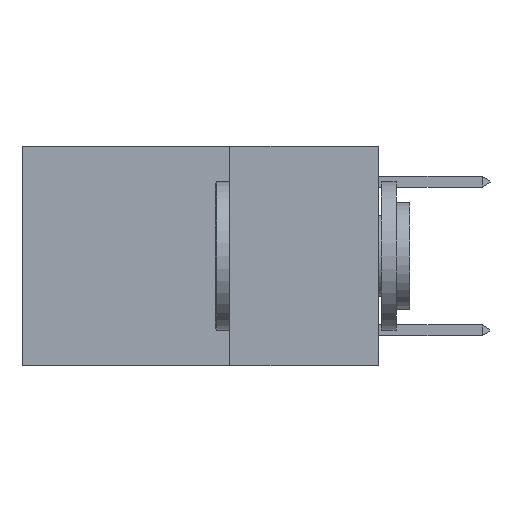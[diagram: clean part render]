
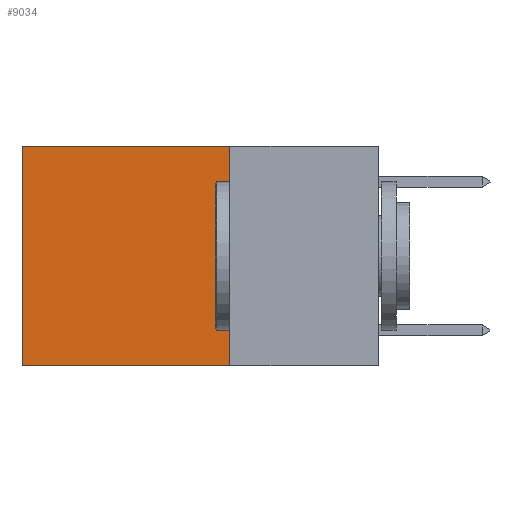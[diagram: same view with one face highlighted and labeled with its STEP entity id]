
A CAD part, left-side view. The second image highlights one B-rep face of the part: STEP entity #9034.
In plain terms, the highlighted planar face has unit normal (-1, 0, 0).
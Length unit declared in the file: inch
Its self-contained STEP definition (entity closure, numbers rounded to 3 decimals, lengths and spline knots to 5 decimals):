
#34 = EDGE_LOOP ( 'NONE', ( #12272, #21927, #20050, #18828 ) ) ;
#1859 = EDGE_CURVE ( 'NONE', #19730, #19976, #15999, .T. ) ;
#3549 = CARTESIAN_POINT ( 'NONE',  ( 0.2625, 0.25, 0. ) ) ;
#3548 = VECTOR ( 'NONE', #12937, 39.37008 ) ;
#3573 = VECTOR ( 'NONE', #8988, 39.37008 ) ;
#3718 = CARTESIAN_POINT ( 'NONE',  ( 0.2625, 0.25, -0.37 ) ) ;
#5790 = CARTESIAN_POINT ( 'NONE',  ( 0.2625, 0.25, -0.37 ) ) ;
#6037 = EDGE_CURVE ( 'NONE', #19730, #17663, #15828, .T. ) ;
#6573 = LINE ( 'NONE', #5790, #3573 ) ;
#7294 = CARTESIAN_POINT ( 'NONE',  ( 0.2625, 0.25, 0. ) ) ;
#7541 = CARTESIAN_POINT ( 'NONE',  ( 0.2625, 0.6, 0. ) ) ;
#8988 = DIRECTION ( 'NONE',  ( 0., 1., 0. ) ) ;
#9015 = LINE ( 'NONE', #9430, #3548 ) ;
#9034 = ADVANCED_FACE ( 'NONE', ( #9570 ), #20997, .F. ) ;
#9430 = CARTESIAN_POINT ( 'NONE',  ( 0.2625, 0.6, 0. ) ) ;
#9570 = FACE_OUTER_BOUND ( 'NONE', #34, .T. ) ;
#9741 = CARTESIAN_POINT ( 'NONE',  ( 0.2625, 0.6, -0.37 ) ) ;
#10288 = EDGE_CURVE ( 'NONE', #17663, #16092, #9015, .T. ) ;
#10631 = DIRECTION ( 'NONE',  ( 0., 0., -1. ) ) ;
#11020 = DIRECTION ( 'NONE',  ( 0., 1., 0. ) ) ;
#11239 = VECTOR ( 'NONE', #11020, 39.37008 ) ;
#12200 = DIRECTION ( 'NONE',  ( 0., 0., -1. ) ) ;
#12272 = ORIENTED_EDGE ( 'NONE', *, *, #10288, .T. ) ;
#12937 = DIRECTION ( 'NONE',  ( 0., 0., -1. ) ) ;
#13463 = CARTESIAN_POINT ( 'NONE',  ( 0.2625, 0.25, 0. ) ) ;
#14540 = AXIS2_PLACEMENT_3D ( 'NONE', #3549, #17423, #10631 ) ;
#15828 = LINE ( 'NONE', #7294, #11239 ) ;
#15999 = LINE ( 'NONE', #18783, #16214 ) ;
#16092 = VERTEX_POINT ( 'NONE', #9741 ) ;
#16214 = VECTOR ( 'NONE', #12200, 39.37008 ) ;
#17423 = DIRECTION ( 'NONE',  ( 1., 0., 0. ) ) ;
#17663 = VERTEX_POINT ( 'NONE', #7541 ) ;
#18783 = CARTESIAN_POINT ( 'NONE',  ( 0.2625, 0.25, 0. ) ) ;
#18828 = ORIENTED_EDGE ( 'NONE', *, *, #6037, .T. ) ;
#19730 = VERTEX_POINT ( 'NONE', #13463 ) ;
#19976 = VERTEX_POINT ( 'NONE', #3718 ) ;
#20050 = ORIENTED_EDGE ( 'NONE', *, *, #1859, .F. ) ;
#20538 = EDGE_CURVE ( 'NONE', #19976, #16092, #6573, .T. ) ;
#20997 = PLANE ( 'NONE',  #14540 ) ;
#21927 = ORIENTED_EDGE ( 'NONE', *, *, #20538, .F. ) ;
